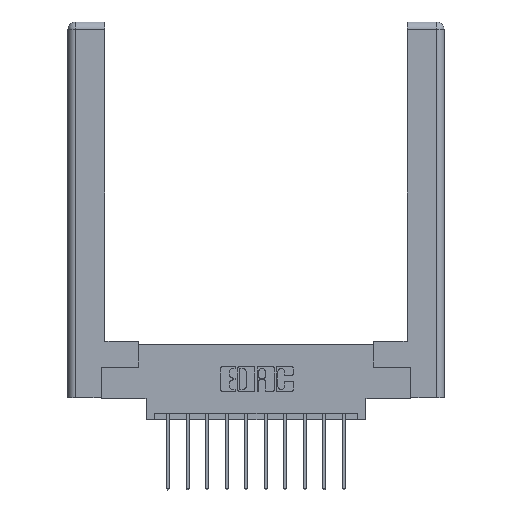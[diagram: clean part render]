
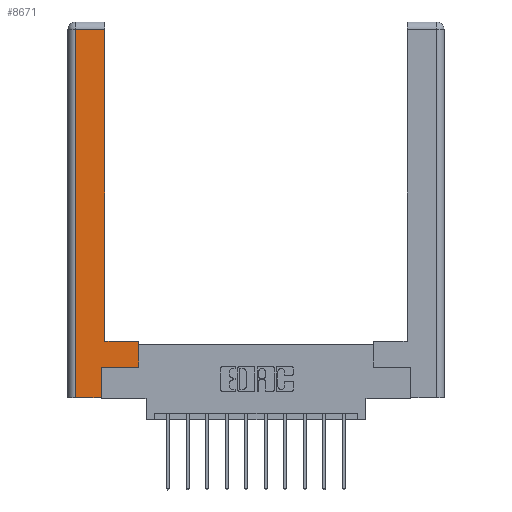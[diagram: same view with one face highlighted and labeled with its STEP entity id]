
A CAD part, top view. The second image highlights one B-rep face of the part: STEP entity #8671.
In plain terms, the highlighted planar face has unit normal (0, 0, 1).
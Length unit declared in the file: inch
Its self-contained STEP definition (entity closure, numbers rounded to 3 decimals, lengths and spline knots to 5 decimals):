
#18 = CARTESIAN_POINT ( 'NONE',  ( 0.265, 0.245, 0. ) ) ;
#70 = VECTOR ( 'NONE', #7348, 39.37008 ) ;
#253 = LINE ( 'NONE', #6208, #70 ) ;
#372 = CARTESIAN_POINT ( 'NONE',  ( 0.565, 0.45, 0. ) ) ;
#393 = VECTOR ( 'NONE', #10996, 39.37008 ) ;
#704 = EDGE_CURVE ( 'NONE', #12754, #13038, #3756, .T. ) ;
#777 = CARTESIAN_POINT ( 'NONE',  ( 0.0615, 0., 0. ) ) ;
#1769 = ORIENTED_EDGE ( 'NONE', *, *, #5816, .T. ) ;
#2225 = EDGE_LOOP ( 'NONE', ( #5802, #12297, #12143, #3752, #1769, #12346, #2819, #9851 ) ) ;
#2798 = CARTESIAN_POINT ( 'NONE',  ( 0.565, 0.245, 0. ) ) ;
#2812 = CARTESIAN_POINT ( 'NONE',  ( 0.565, 0.245, 0. ) ) ;
#2819 = ORIENTED_EDGE ( 'NONE', *, *, #6662, .T. ) ;
#2935 = LINE ( 'NONE', #4576, #11259 ) ;
#3211 = CARTESIAN_POINT ( 'NONE',  ( 0.265, 0.245, 0. ) ) ;
#3222 = CARTESIAN_POINT ( 'NONE',  ( 0.295, 0.45, 0. ) ) ;
#3273 = DIRECTION ( 'NONE',  ( -1., 0., 0. ) ) ;
#3406 = CARTESIAN_POINT ( 'NONE',  ( 0.0615, 0., 0. ) ) ;
#3553 = DIRECTION ( 'NONE',  ( 0., 0., -1. ) ) ;
#3752 = ORIENTED_EDGE ( 'NONE', *, *, #8638, .T. ) ;
#3756 = LINE ( 'NONE', #777, #393 ) ;
#4040 = VERTEX_POINT ( 'NONE', #372 ) ;
#4269 = VERTEX_POINT ( 'NONE', #9613 ) ;
#4523 = PLANE ( 'NONE',  #13123 ) ;
#4576 = CARTESIAN_POINT ( 'NONE',  ( 0.265, 0., 0. ) ) ;
#4696 = CARTESIAN_POINT ( 'NONE',  ( 0.295, 0.45, 0. ) ) ;
#4712 = VECTOR ( 'NONE', #10111, 39.37008 ) ;
#5287 = VECTOR ( 'NONE', #6701, 39.37008 ) ;
#5304 = VERTEX_POINT ( 'NONE', #18 ) ;
#5677 = CARTESIAN_POINT ( 'NONE',  ( 0.265, 0., 0. ) ) ;
#5802 = ORIENTED_EDGE ( 'NONE', *, *, #8060, .T. ) ;
#5816 = EDGE_CURVE ( 'NONE', #8180, #5304, #8481, .T. ) ;
#5961 = FACE_OUTER_BOUND ( 'NONE', #2225, .T. ) ;
#6208 = CARTESIAN_POINT ( 'NONE',  ( 0.0615, 2.94, 0. ) ) ;
#6662 = EDGE_CURVE ( 'NONE', #14695, #4040, #14351, .T. ) ;
#6701 = DIRECTION ( 'NONE',  ( 0., 1., 0. ) ) ;
#6784 = VECTOR ( 'NONE', #9549, 39.37008 ) ;
#6871 = DIRECTION ( 'NONE',  ( -1., 0., 0. ) ) ;
#7348 = DIRECTION ( 'NONE',  ( -1., 0., 0. ) ) ;
#7931 = VECTOR ( 'NONE', #3273, 39.37008 ) ;
#8060 = EDGE_CURVE ( 'NONE', #14361, #4269, #8067, .T. ) ;
#8067 = LINE ( 'NONE', #12112, #4712 ) ;
#8175 = LINE ( 'NONE', #2798, #6784 ) ;
#8180 = VERTEX_POINT ( 'NONE', #5677 ) ;
#8481 = LINE ( 'NONE', #3211, #10785 ) ;
#8638 = EDGE_CURVE ( 'NONE', #13038, #8180, #2935, .T. ) ;
#8671 = ADVANCED_FACE ( 'NONE', ( #5961 ), #4523, .F. ) ;
#9549 = DIRECTION ( 'NONE',  ( 1., 0., 0. ) ) ;
#9613 = CARTESIAN_POINT ( 'NONE',  ( 0.295, 2.94, 0. ) ) ;
#9851 = ORIENTED_EDGE ( 'NONE', *, *, #14263, .T. ) ;
#10111 = DIRECTION ( 'NONE',  ( 0., 1., 0. ) ) ;
#10269 = CARTESIAN_POINT ( 'NONE',  ( 0., 0., 0. ) ) ;
#10290 = EDGE_CURVE ( 'NONE', #5304, #14695, #8175, .T. ) ;
#10415 = LINE ( 'NONE', #3222, #7931 ) ;
#10785 = VECTOR ( 'NONE', #10968, 39.37008 ) ;
#10910 = EDGE_CURVE ( 'NONE', #4269, #12754, #253, .T. ) ;
#10968 = DIRECTION ( 'NONE',  ( 0., 1., 0. ) ) ;
#10996 = DIRECTION ( 'NONE',  ( 0., -1., 0. ) ) ;
#11259 = VECTOR ( 'NONE', #12518, 39.37008 ) ;
#12112 = CARTESIAN_POINT ( 'NONE',  ( 0.295, 3., 0. ) ) ;
#12143 = ORIENTED_EDGE ( 'NONE', *, *, #704, .T. ) ;
#12149 = CARTESIAN_POINT ( 'NONE',  ( 0.565, 0.45, 0. ) ) ;
#12297 = ORIENTED_EDGE ( 'NONE', *, *, #10910, .T. ) ;
#12346 = ORIENTED_EDGE ( 'NONE', *, *, #10290, .T. ) ;
#12518 = DIRECTION ( 'NONE',  ( 1., 0., 0. ) ) ;
#12754 = VERTEX_POINT ( 'NONE', #14229 ) ;
#13038 = VERTEX_POINT ( 'NONE', #3406 ) ;
#13123 = AXIS2_PLACEMENT_3D ( 'NONE', #10269, #3553, #6871 ) ;
#14229 = CARTESIAN_POINT ( 'NONE',  ( 0.0615, 2.94, 0. ) ) ;
#14263 = EDGE_CURVE ( 'NONE', #4040, #14361, #10415, .T. ) ;
#14351 = LINE ( 'NONE', #12149, #5287 ) ;
#14361 = VERTEX_POINT ( 'NONE', #4696 ) ;
#14695 = VERTEX_POINT ( 'NONE', #2812 ) ;
